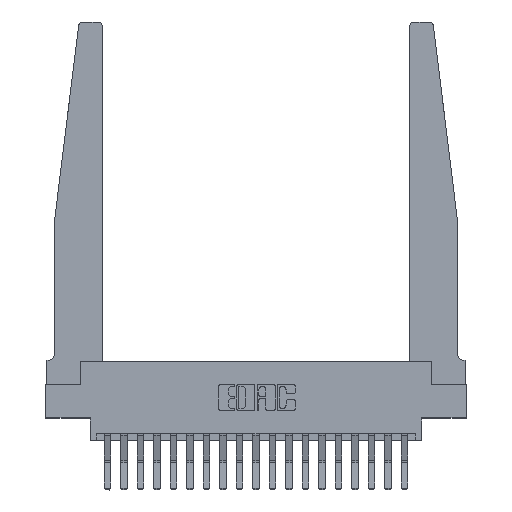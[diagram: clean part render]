
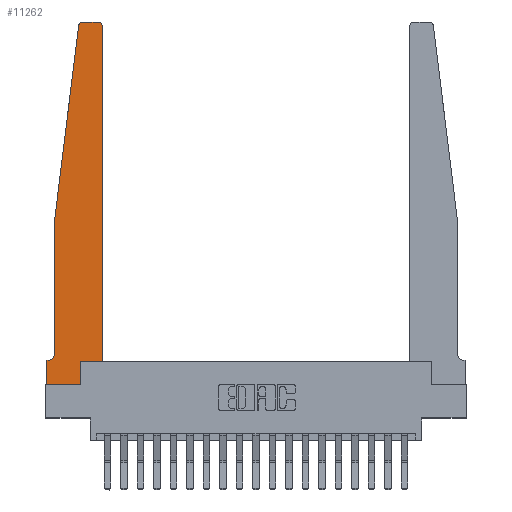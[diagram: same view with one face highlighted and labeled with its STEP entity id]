
A CAD part, top view. The second image highlights one B-rep face of the part: STEP entity #11262.
In plain terms, the highlighted planar face has unit normal (0, 0, 1).
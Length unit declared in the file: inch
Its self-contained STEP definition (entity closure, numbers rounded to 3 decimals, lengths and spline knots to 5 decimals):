
#130 = DIRECTION ( 'NONE',  ( -1., 0., 0. ) ) ;
#167 = FACE_OUTER_BOUND ( 'NONE', #18468, .T. ) ;
#177 = ORIENTED_EDGE ( 'NONE', *, *, #14184, .T. ) ;
#388 = CARTESIAN_POINT ( 'NONE',  ( 0.395, 2.72, 0.37 ) ) ;
#837 = EDGE_CURVE ( 'NONE', #8972, #9691, #10825, .T. ) ;
#909 = VERTEX_POINT ( 'NONE', #4861 ) ;
#1222 = VECTOR ( 'NONE', #19014, 39.37008 ) ;
#1994 = DIRECTION ( 'NONE',  ( 1., 0., 0. ) ) ;
#2116 = VERTEX_POINT ( 'NONE', #11507 ) ;
#2247 = EDGE_CURVE ( 'NONE', #4035, #20214, #8040, .T. ) ;
#2438 = ORIENTED_EDGE ( 'NONE', *, *, #15074, .T. ) ;
#2474 = CIRCLE ( 'NONE', #14967, 0.03 ) ;
#2644 = CARTESIAN_POINT ( 'NONE',  ( 0.425, 0.18, 0.37 ) ) ;
#2909 = DIRECTION ( 'NONE',  ( 0., -1., 0. ) ) ;
#3120 = CARTESIAN_POINT ( 'NONE',  ( 0.2605, 0.18, 0.37 ) ) ;
#3266 = CIRCLE ( 'NONE', #4748, 0.05 ) ;
#3370 = VERTEX_POINT ( 'NONE', #18073 ) ;
#3409 = LINE ( 'NONE', #14055, #7147 ) ;
#4035 = VERTEX_POINT ( 'NONE', #15399 ) ;
#4214 = ORIENTED_EDGE ( 'NONE', *, *, #5467, .T. ) ;
#4416 = CARTESIAN_POINT ( 'NONE',  ( 0.2605, 0., 0.37 ) ) ;
#4422 = PLANE ( 'NONE',  #16267 ) ;
#4544 = DIRECTION ( 'NONE',  ( 0., 0., 1. ) ) ;
#4557 = VECTOR ( 'NONE', #11036, 39.37008 ) ;
#4748 = AXIS2_PLACEMENT_3D ( 'NONE', #17534, #8046, #19113 ) ;
#4787 = CARTESIAN_POINT ( 'NONE',  ( 0., 0.1875, 0.37 ) ) ;
#4861 = CARTESIAN_POINT ( 'NONE',  ( 0., 0., 0.37 ) ) ;
#5006 = LINE ( 'NONE', #6430, #12497 ) ;
#5096 = CARTESIAN_POINT ( 'NONE',  ( 0.2605, 0.18, 0.37 ) ) ;
#5231 = EDGE_CURVE ( 'NONE', #2116, #10962, #2474, .T. ) ;
#5324 = CARTESIAN_POINT ( 'NONE',  ( 0.24675, 2.72367, 0.37 ) ) ;
#5421 = CARTESIAN_POINT ( 'NONE',  ( 0.065, 1.25, 0.37 ) ) ;
#5467 = EDGE_CURVE ( 'NONE', #17354, #10388, #19563, .T. ) ;
#5568 = LINE ( 'NONE', #15146, #13580 ) ;
#5962 = CARTESIAN_POINT ( 'NONE',  ( 0.425, 0.18, 0.37 ) ) ;
#6202 = VECTOR ( 'NONE', #18638, 39.37008 ) ;
#6319 = CARTESIAN_POINT ( 'NONE',  ( 0.425, 0.18, 0.37 ) ) ;
#6430 = CARTESIAN_POINT ( 'NONE',  ( 0.25, 2.75, 0.37 ) ) ;
#6524 = EDGE_CURVE ( 'NONE', #19203, #909, #3409, .T. ) ;
#6695 = ORIENTED_EDGE ( 'NONE', *, *, #837, .T. ) ;
#7147 = VECTOR ( 'NONE', #2909, 39.37008 ) ;
#7222 = DIRECTION ( 'NONE',  ( -1., 0., 0. ) ) ;
#7536 = VECTOR ( 'NONE', #10255, 39.37008 ) ;
#7624 = DIRECTION ( 'NONE',  ( 0., 0., 1. ) ) ;
#7796 = ORIENTED_EDGE ( 'NONE', *, *, #6524, .T. ) ;
#8040 = LINE ( 'NONE', #5421, #7536 ) ;
#8046 = DIRECTION ( 'NONE',  ( 0., 0., -1. ) ) ;
#8201 = EDGE_CURVE ( 'NONE', #3370, #19203, #5568, .T. ) ;
#8435 = CARTESIAN_POINT ( 'NONE',  ( 0.395, 2.75, 0.37 ) ) ;
#8890 = ORIENTED_EDGE ( 'NONE', *, *, #8201, .T. ) ;
#8955 = EDGE_CURVE ( 'NONE', #10962, #4035, #14683, .T. ) ;
#8972 = VERTEX_POINT ( 'NONE', #4416 ) ;
#9336 = LINE ( 'NONE', #18880, #4557 ) ;
#9388 = ORIENTED_EDGE ( 'NONE', *, *, #13674, .T. ) ;
#9691 = VERTEX_POINT ( 'NONE', #5096 ) ;
#10220 = EDGE_CURVE ( 'NONE', #14114, #17354, #18074, .T. ) ;
#10255 = DIRECTION ( 'NONE',  ( 0., -1., 0. ) ) ;
#10388 = VERTEX_POINT ( 'NONE', #8435 ) ;
#10825 = LINE ( 'NONE', #3120, #14536 ) ;
#10962 = VERTEX_POINT ( 'NONE', #5324 ) ;
#11036 = DIRECTION ( 'NONE',  ( 1., 0., 0. ) ) ;
#11086 = DIRECTION ( 'NONE',  ( 0., 1., 0. ) ) ;
#11262 = ADVANCED_FACE ( 'NONE', ( #167 ), #4422, .T. ) ;
#11507 = CARTESIAN_POINT ( 'NONE',  ( 0.27653, 2.75, 0.37 ) ) ;
#11519 = DIRECTION ( 'NONE',  ( 0., 0., 1. ) ) ;
#12497 = VECTOR ( 'NONE', #130, 39.37008 ) ;
#12530 = VECTOR ( 'NONE', #15505, 39.37008 ) ;
#12860 = CARTESIAN_POINT ( 'NONE',  ( 0.065, 0.2375, 0.37 ) ) ;
#13580 = VECTOR ( 'NONE', #7222, 39.37008 ) ;
#13674 = EDGE_CURVE ( 'NONE', #909, #8972, #9336, .T. ) ;
#14055 = CARTESIAN_POINT ( 'NONE',  ( 0., 0., 0.37 ) ) ;
#14110 = CARTESIAN_POINT ( 'NONE',  ( 0.27653, 2.72, 0.37 ) ) ;
#14114 = VERTEX_POINT ( 'NONE', #2644 ) ;
#14184 = EDGE_CURVE ( 'NONE', #9691, #14114, #20387, .T. ) ;
#14536 = VECTOR ( 'NONE', #11086, 39.37008 ) ;
#14683 = LINE ( 'NONE', #20127, #6202 ) ;
#14761 = ORIENTED_EDGE ( 'NONE', *, *, #2247, .T. ) ;
#14925 = EDGE_CURVE ( 'NONE', #20214, #3370, #3266, .T. ) ;
#14967 = AXIS2_PLACEMENT_3D ( 'NONE', #14110, #4544, #15675 ) ;
#15074 = EDGE_CURVE ( 'NONE', #10388, #2116, #5006, .T. ) ;
#15146 = CARTESIAN_POINT ( 'NONE',  ( 0.065, 0.1875, 0.37 ) ) ;
#15399 = CARTESIAN_POINT ( 'NONE',  ( 0.065, 1.25, 0.37 ) ) ;
#15505 = DIRECTION ( 'NONE',  ( 1., 0., 0. ) ) ;
#15675 = DIRECTION ( 'NONE',  ( 1., 0., 0. ) ) ;
#16267 = AXIS2_PLACEMENT_3D ( 'NONE', #17120, #7624, #18709 ) ;
#16663 = ORIENTED_EDGE ( 'NONE', *, *, #10220, .T. ) ;
#16970 = ORIENTED_EDGE ( 'NONE', *, *, #8955, .T. ) ;
#17120 = CARTESIAN_POINT ( 'NONE',  ( 0., 0.1875, 0.37 ) ) ;
#17175 = CARTESIAN_POINT ( 'NONE',  ( 0.425, 2.72, 0.37 ) ) ;
#17354 = VERTEX_POINT ( 'NONE', #17175 ) ;
#17534 = CARTESIAN_POINT ( 'NONE',  ( 0.015, 0.2375, 0.37 ) ) ;
#18073 = CARTESIAN_POINT ( 'NONE',  ( 0.015, 0.1875, 0.37 ) ) ;
#18074 = LINE ( 'NONE', #6319, #1222 ) ;
#18468 = EDGE_LOOP ( 'NONE', ( #2438, #20310, #16970, #14761, #18998, #8890, #7796, #9388, #6695, #177, #16663, #4214 ) ) ;
#18638 = DIRECTION ( 'NONE',  ( -0.122, -0.992, 0. ) ) ;
#18709 = DIRECTION ( 'NONE',  ( 1., 0., 0. ) ) ;
#18880 = CARTESIAN_POINT ( 'NONE',  ( 0., 0., 0.37 ) ) ;
#18998 = ORIENTED_EDGE ( 'NONE', *, *, #14925, .T. ) ;
#19014 = DIRECTION ( 'NONE',  ( 0., 1., 0. ) ) ;
#19113 = DIRECTION ( 'NONE',  ( -1., 0., 0. ) ) ;
#19203 = VERTEX_POINT ( 'NONE', #4787 ) ;
#19563 = CIRCLE ( 'NONE', #19757, 0.03 ) ;
#19757 = AXIS2_PLACEMENT_3D ( 'NONE', #388, #11519, #1994 ) ;
#20127 = CARTESIAN_POINT ( 'NONE',  ( 0.065, 1.25, 0.37 ) ) ;
#20214 = VERTEX_POINT ( 'NONE', #12860 ) ;
#20310 = ORIENTED_EDGE ( 'NONE', *, *, #5231, .T. ) ;
#20387 = LINE ( 'NONE', #5962, #12530 ) ;
